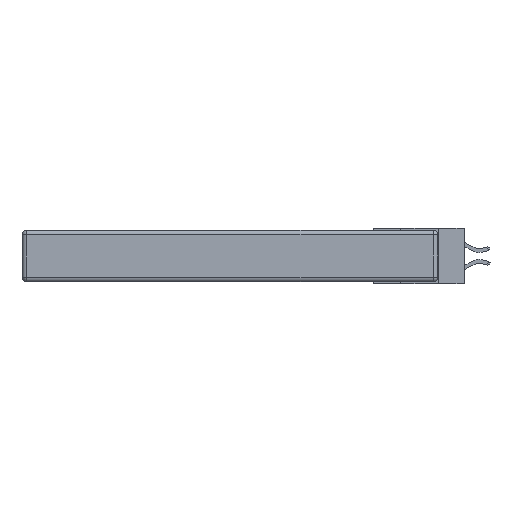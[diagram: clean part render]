
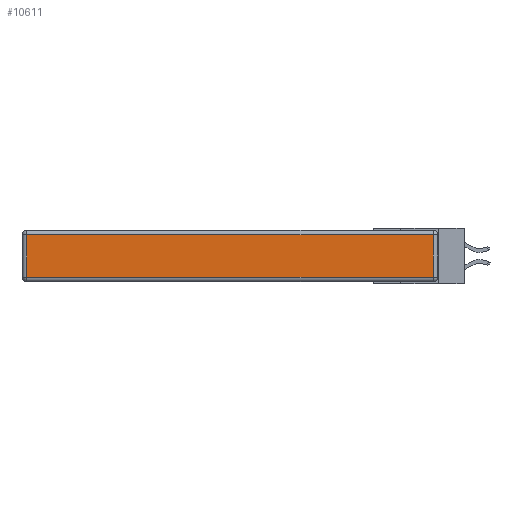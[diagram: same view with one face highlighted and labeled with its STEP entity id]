
A CAD part, left-side view. The second image highlights one B-rep face of the part: STEP entity #10611.
In plain terms, the highlighted planar face has unit normal (-1, 0, 0).
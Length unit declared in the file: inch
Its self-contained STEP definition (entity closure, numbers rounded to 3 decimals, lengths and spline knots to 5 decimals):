
#523 = DIRECTION ( 'NONE',  ( 0., 0., 1. ) ) ;
#846 = VECTOR ( 'NONE', #11213, 39.37008 ) ;
#1121 = ORIENTED_EDGE ( 'NONE', *, *, #10350, .T. ) ;
#1714 = ORIENTED_EDGE ( 'NONE', *, *, #5775, .T. ) ;
#1845 = LINE ( 'NONE', #2259, #12478 ) ;
#1918 = AXIS2_PLACEMENT_3D ( 'NONE', #14383, #17609, #11239 ) ;
#2259 = CARTESIAN_POINT ( 'NONE',  ( 0., 0.03, -0.343 ) ) ;
#3319 = DIRECTION ( 'NONE',  ( 0., -1., 0. ) ) ;
#3667 = CARTESIAN_POINT ( 'NONE',  ( 0., 2.72, -0.03 ) ) ;
#5775 = EDGE_CURVE ( 'NONE', #15984, #9398, #19430, .T. ) ;
#5973 = VERTEX_POINT ( 'NONE', #9076 ) ;
#6602 = LINE ( 'NONE', #9433, #846 ) ;
#7123 = VERTEX_POINT ( 'NONE', #3667 ) ;
#7700 = CARTESIAN_POINT ( 'NONE',  ( 0., 0.03, -0.313 ) ) ;
#7770 = CARTESIAN_POINT ( 'NONE',  ( 0., 0., -0.313 ) ) ;
#8435 = LINE ( 'NONE', #17455, #14007 ) ;
#9076 = CARTESIAN_POINT ( 'NONE',  ( 0., 0.03, -0.03 ) ) ;
#9398 = VERTEX_POINT ( 'NONE', #7700 ) ;
#9433 = CARTESIAN_POINT ( 'NONE',  ( 0., 2.72, -0.343 ) ) ;
#9604 = EDGE_CURVE ( 'NONE', #5973, #7123, #8435, .T. ) ;
#9741 = PLANE ( 'NONE',  #1918 ) ;
#9894 = VECTOR ( 'NONE', #3319, 39.37008 ) ;
#10350 = EDGE_CURVE ( 'NONE', #9398, #5973, #1845, .T. ) ;
#10611 = ADVANCED_FACE ( 'NONE', ( #15458 ), #9741, .T. ) ;
#10832 = EDGE_LOOP ( 'NONE', ( #1714, #1121, #19007, #19514 ) ) ;
#10946 = EDGE_CURVE ( 'NONE', #7123, #15984, #6602, .T. ) ;
#11009 = CARTESIAN_POINT ( 'NONE',  ( 0., 2.72, -0.313 ) ) ;
#11213 = DIRECTION ( 'NONE',  ( 0., 0., -1. ) ) ;
#11239 = DIRECTION ( 'NONE',  ( 0., 0., 1. ) ) ;
#12478 = VECTOR ( 'NONE', #523, 39.37008 ) ;
#14007 = VECTOR ( 'NONE', #15673, 39.37008 ) ;
#14383 = CARTESIAN_POINT ( 'NONE',  ( 0., 0., -0.343 ) ) ;
#15458 = FACE_OUTER_BOUND ( 'NONE', #10832, .T. ) ;
#15673 = DIRECTION ( 'NONE',  ( 0., 1., 0. ) ) ;
#15984 = VERTEX_POINT ( 'NONE', #11009 ) ;
#17455 = CARTESIAN_POINT ( 'NONE',  ( 0., 2.75, -0.03 ) ) ;
#17609 = DIRECTION ( 'NONE',  ( -1., 0., 0. ) ) ;
#19007 = ORIENTED_EDGE ( 'NONE', *, *, #9604, .T. ) ;
#19430 = LINE ( 'NONE', #7770, #9894 ) ;
#19514 = ORIENTED_EDGE ( 'NONE', *, *, #10946, .T. ) ;
